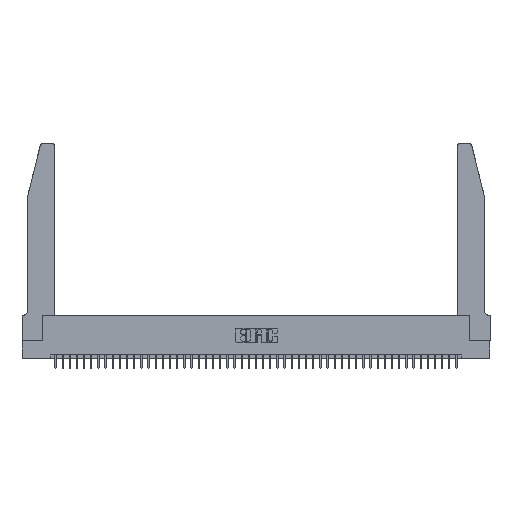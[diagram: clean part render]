
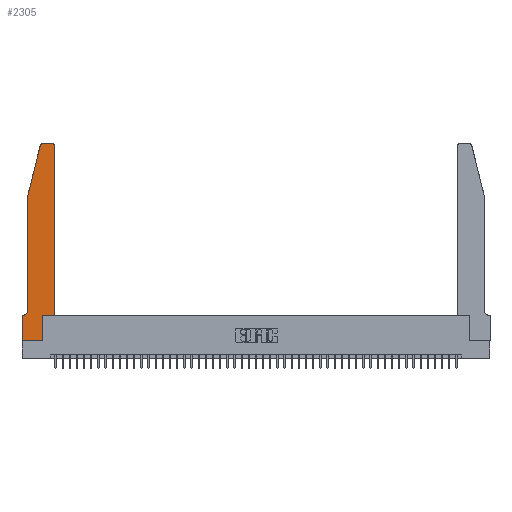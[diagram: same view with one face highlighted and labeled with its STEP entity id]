
A CAD part, top view. The second image highlights one B-rep face of the part: STEP entity #2305.
In plain terms, the highlighted planar face has unit normal (0, 0, 1).
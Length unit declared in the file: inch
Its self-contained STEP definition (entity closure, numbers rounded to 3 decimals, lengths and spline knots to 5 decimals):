
#560 = ORIENTED_EDGE ( 'NONE', *, *, #17650, .T. ) ;
#2117 = DIRECTION ( 'NONE',  ( -0.239, -0.971, 0. ) ) ;
#2305 = ADVANCED_FACE ( 'NONE', ( #32644 ), #10357, .T. ) ;
#2695 = ORIENTED_EDGE ( 'NONE', *, *, #37460, .T. ) ;
#2714 = VECTOR ( 'NONE', #39008, 39.37008 ) ;
#2745 = DIRECTION ( 'NONE',  ( 1., 0., 0. ) ) ;
#2795 = ORIENTED_EDGE ( 'NONE', *, *, #5038, .T. ) ;
#2862 = ORIENTED_EDGE ( 'NONE', *, *, #45401, .T. ) ;
#3433 = CIRCLE ( 'NONE', #21134, 0.03 ) ;
#3524 = VERTEX_POINT ( 'NONE', #12571 ) ;
#4250 = CARTESIAN_POINT ( 'NONE',  ( 0.2865, 0.35, 0.37 ) ) ;
#4942 = VERTEX_POINT ( 'NONE', #15271 ) ;
#5038 = EDGE_CURVE ( 'NONE', #18560, #39200, #37820, .T. ) ;
#5185 = CARTESIAN_POINT ( 'NONE',  ( 0.4205, 2.72, 0.37 ) ) ;
#6124 = ORIENTED_EDGE ( 'NONE', *, *, #24364, .T. ) ;
#6678 = ORIENTED_EDGE ( 'NONE', *, *, #29567, .T. ) ;
#6734 = CARTESIAN_POINT ( 'NONE',  ( 0., 0., 0.37 ) ) ;
#6816 = EDGE_CURVE ( 'NONE', #39200, #24185, #19125, .T. ) ;
#8513 = CARTESIAN_POINT ( 'NONE',  ( 0.4505, 0.35, 0.37 ) ) ;
#9173 = EDGE_CURVE ( 'NONE', #26887, #32466, #36223, .T. ) ;
#9600 = LINE ( 'NONE', #34819, #16504 ) ;
#10357 = PLANE ( 'NONE',  #41482 ) ;
#10391 = VECTOR ( 'NONE', #32698, 39.37008 ) ;
#10561 = ORIENTED_EDGE ( 'NONE', *, *, #6816, .T. ) ;
#11742 = DIRECTION ( 'NONE',  ( 0., 1., 0. ) ) ;
#11797 = ORIENTED_EDGE ( 'NONE', *, *, #47403, .T. ) ;
#12571 = CARTESIAN_POINT ( 'NONE',  ( 0.25487, 2.72718, 0.37 ) ) ;
#13477 = DIRECTION ( 'NONE',  ( 0., 0., 1. ) ) ;
#13758 = DIRECTION ( 'NONE',  ( 0., -1., 0. ) ) ;
#13805 = DIRECTION ( 'NONE',  ( 0., 0., -1. ) ) ;
#14235 = CARTESIAN_POINT ( 'NONE',  ( 0.0755, 2., 0.37 ) ) ;
#14268 = EDGE_LOOP ( 'NONE', ( #6124, #34503, #37881, #6678, #11797, #14809, #2695, #560, #2862, #40582, #2795, #10561 ) ) ;
#14317 = CARTESIAN_POINT ( 'NONE',  ( 0.284, 2.75, 0.37 ) ) ;
#14745 = VERTEX_POINT ( 'NONE', #14317 ) ;
#14809 = ORIENTED_EDGE ( 'NONE', *, *, #9173, .T. ) ;
#15271 = CARTESIAN_POINT ( 'NONE',  ( 0., 0., 0.37 ) ) ;
#15616 = VERTEX_POINT ( 'NONE', #29471 ) ;
#16461 = LINE ( 'NONE', #28420, #2714 ) ;
#16504 = VECTOR ( 'NONE', #2117, 39.37008 ) ;
#16728 = VECTOR ( 'NONE', #26772, 39.37008 ) ;
#17396 = CARTESIAN_POINT ( 'NONE',  ( 0.0055, 0.42, 0.37 ) ) ;
#17504 = DIRECTION ( 'NONE',  ( -1., 0., 0. ) ) ;
#17650 = EDGE_CURVE ( 'NONE', #4942, #30930, #34547, .T. ) ;
#17827 = LINE ( 'NONE', #6734, #25461 ) ;
#18560 = VERTEX_POINT ( 'NONE', #23265 ) ;
#19125 = CIRCLE ( 'NONE', #37541, 0.03 ) ;
#19339 = VECTOR ( 'NONE', #42770, 39.37008 ) ;
#19865 = DIRECTION ( 'NONE',  ( 1., 0., 0. ) ) ;
#19902 = CARTESIAN_POINT ( 'NONE',  ( 0., 0., 0.37 ) ) ;
#20640 = LINE ( 'NONE', #35293, #19339 ) ;
#21134 = AXIS2_PLACEMENT_3D ( 'NONE', #39310, #32080, #2745 ) ;
#22801 = CARTESIAN_POINT ( 'NONE',  ( 0.0055, 0.35, 0.37 ) ) ;
#23265 = CARTESIAN_POINT ( 'NONE',  ( 0.4505, 0.35, 0.37 ) ) ;
#23391 = CARTESIAN_POINT ( 'NONE',  ( 0.0755, 2., 0.37 ) ) ;
#24185 = VERTEX_POINT ( 'NONE', #40143 ) ;
#24364 = EDGE_CURVE ( 'NONE', #24185, #14745, #20640, .T. ) ;
#25068 = CIRCLE ( 'NONE', #31221, 0.07 ) ;
#25461 = VECTOR ( 'NONE', #13758, 39.37008 ) ;
#26477 = CARTESIAN_POINT ( 'NONE',  ( 0.2865, 0., 0.37 ) ) ;
#26772 = DIRECTION ( 'NONE',  ( 0., 1., 0. ) ) ;
#26887 = VERTEX_POINT ( 'NONE', #22801 ) ;
#28420 = CARTESIAN_POINT ( 'NONE',  ( 0.4505, 0.35, 0.37 ) ) ;
#29471 = CARTESIAN_POINT ( 'NONE',  ( 0.0755, 0.42, 0.37 ) ) ;
#29567 = EDGE_CURVE ( 'NONE', #38576, #15616, #47195, .T. ) ;
#30099 = VECTOR ( 'NONE', #30938, 39.37008 ) ;
#30930 = VERTEX_POINT ( 'NONE', #26477 ) ;
#30938 = DIRECTION ( 'NONE',  ( 1., 0., 0. ) ) ;
#31221 = AXIS2_PLACEMENT_3D ( 'NONE', #17396, #13805, #43124 ) ;
#31714 = CARTESIAN_POINT ( 'NONE',  ( 0., 0.35, 0.37 ) ) ;
#32080 = DIRECTION ( 'NONE',  ( 0., 0., 1. ) ) ;
#32466 = VERTEX_POINT ( 'NONE', #37262 ) ;
#32644 = FACE_OUTER_BOUND ( 'NONE', #14268, .T. ) ;
#32698 = DIRECTION ( 'NONE',  ( 0., -1., 0. ) ) ;
#32846 = CARTESIAN_POINT ( 'NONE',  ( 0.0755, 0.35, 0.37 ) ) ;
#34503 = ORIENTED_EDGE ( 'NONE', *, *, #43436, .T. ) ;
#34547 = LINE ( 'NONE', #19902, #30099 ) ;
#34819 = CARTESIAN_POINT ( 'NONE',  ( 0.0755, 2., 0.37 ) ) ;
#35293 = CARTESIAN_POINT ( 'NONE',  ( 0.2605, 2.75, 0.37 ) ) ;
#35708 = VECTOR ( 'NONE', #11742, 39.37008 ) ;
#36223 = LINE ( 'NONE', #32846, #43548 ) ;
#36448 = LINE ( 'NONE', #4250, #35708 ) ;
#37262 = CARTESIAN_POINT ( 'NONE',  ( 0., 0.35, 0.37 ) ) ;
#37460 = EDGE_CURVE ( 'NONE', #32466, #4942, #17827, .T. ) ;
#37541 = AXIS2_PLACEMENT_3D ( 'NONE', #5185, #38343, #19865 ) ;
#37820 = LINE ( 'NONE', #8513, #16728 ) ;
#37881 = ORIENTED_EDGE ( 'NONE', *, *, #42800, .T. ) ;
#38343 = DIRECTION ( 'NONE',  ( 0., 0., 1. ) ) ;
#38576 = VERTEX_POINT ( 'NONE', #23391 ) ;
#39008 = DIRECTION ( 'NONE',  ( 1., 0., 0. ) ) ;
#39200 = VERTEX_POINT ( 'NONE', #43984 ) ;
#39310 = CARTESIAN_POINT ( 'NONE',  ( 0.284, 2.72, 0.37 ) ) ;
#40143 = CARTESIAN_POINT ( 'NONE',  ( 0.4205, 2.75, 0.37 ) ) ;
#40582 = ORIENTED_EDGE ( 'NONE', *, *, #45974, .T. ) ;
#41482 = AXIS2_PLACEMENT_3D ( 'NONE', #31714, #13477, #42804 ) ;
#42770 = DIRECTION ( 'NONE',  ( -1., 0., 0. ) ) ;
#42800 = EDGE_CURVE ( 'NONE', #3524, #38576, #9600, .T. ) ;
#42804 = DIRECTION ( 'NONE',  ( 1., 0., 0. ) ) ;
#43124 = DIRECTION ( 'NONE',  ( -1., 0., 0. ) ) ;
#43436 = EDGE_CURVE ( 'NONE', #14745, #3524, #3433, .T. ) ;
#43548 = VECTOR ( 'NONE', #17504, 39.37008 ) ;
#43591 = CARTESIAN_POINT ( 'NONE',  ( 0.2865, 0.35, 0.37 ) ) ;
#43984 = CARTESIAN_POINT ( 'NONE',  ( 0.4505, 2.72, 0.37 ) ) ;
#44350 = VERTEX_POINT ( 'NONE', #43591 ) ;
#45401 = EDGE_CURVE ( 'NONE', #30930, #44350, #36448, .T. ) ;
#45974 = EDGE_CURVE ( 'NONE', #44350, #18560, #16461, .T. ) ;
#47195 = LINE ( 'NONE', #14235, #10391 ) ;
#47403 = EDGE_CURVE ( 'NONE', #15616, #26887, #25068, .T. ) ;
